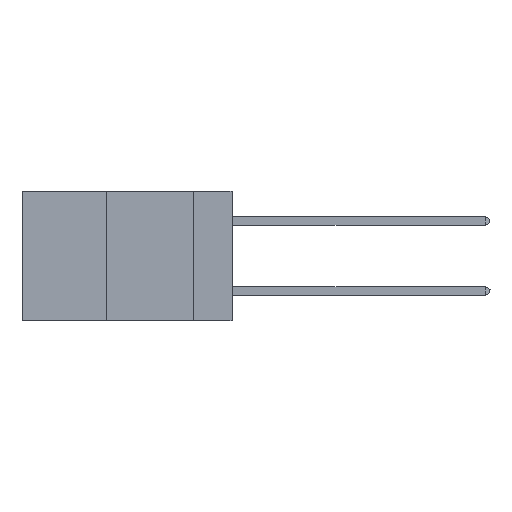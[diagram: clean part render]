
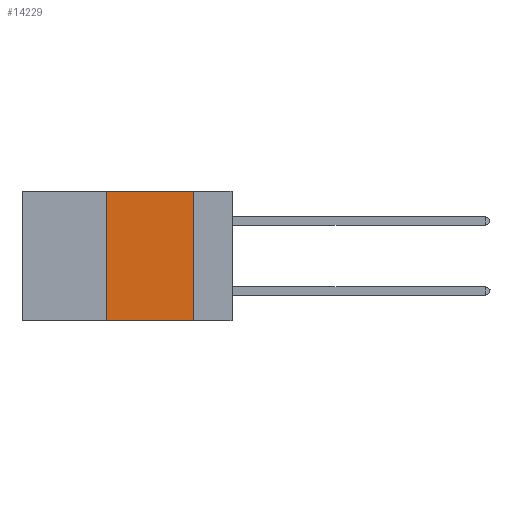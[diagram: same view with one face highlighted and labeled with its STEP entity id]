
A CAD part, left-side view. The second image highlights one B-rep face of the part: STEP entity #14229.
In plain terms, the highlighted planar face has unit normal (-1, 0, 0).
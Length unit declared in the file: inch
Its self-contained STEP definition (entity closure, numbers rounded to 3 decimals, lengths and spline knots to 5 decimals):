
#231 = DIRECTION ( 'NONE',  ( 0., -1., 0. ) ) ;
#595 = CARTESIAN_POINT ( 'NONE',  ( 0., 0.36, -0.37 ) ) ;
#899 = CARTESIAN_POINT ( 'NONE',  ( 0., 0.11, 0. ) ) ;
#1291 = DIRECTION ( 'NONE',  ( 0., 0., 1. ) ) ;
#1660 = VERTEX_POINT ( 'NONE', #8395 ) ;
#2934 = LINE ( 'NONE', #7076, #9794 ) ;
#3061 = EDGE_CURVE ( 'NONE', #1660, #17564, #10608, .T. ) ;
#4936 = CARTESIAN_POINT ( 'NONE',  ( 0., 0.36, 0. ) ) ;
#5480 = LINE ( 'NONE', #14958, #6207 ) ;
#6207 = VECTOR ( 'NONE', #12471, 39.37008 ) ;
#6398 = DIRECTION ( 'NONE',  ( 0., 0., -1. ) ) ;
#6500 = DIRECTION ( 'NONE',  ( 1., 0., 0. ) ) ;
#7076 = CARTESIAN_POINT ( 'NONE',  ( 0., 0.6, -0.37 ) ) ;
#7523 = ORIENTED_EDGE ( 'NONE', *, *, #7615, .T. ) ;
#7615 = EDGE_CURVE ( 'NONE', #10805, #17564, #2934, .T. ) ;
#7930 = FACE_OUTER_BOUND ( 'NONE', #8690, .T. ) ;
#8210 = LINE ( 'NONE', #10807, #11581 ) ;
#8395 = CARTESIAN_POINT ( 'NONE',  ( 0., 0.11, 0. ) ) ;
#8690 = EDGE_LOOP ( 'NONE', ( #16085, #14209, #10103, #7523 ) ) ;
#9794 = VECTOR ( 'NONE', #231, 39.37008 ) ;
#10103 = ORIENTED_EDGE ( 'NONE', *, *, #12572, .F. ) ;
#10608 = LINE ( 'NONE', #899, #15572 ) ;
#10805 = VERTEX_POINT ( 'NONE', #595 ) ;
#10807 = CARTESIAN_POINT ( 'NONE',  ( 0., 0.36, 0. ) ) ;
#10818 = CARTESIAN_POINT ( 'NONE',  ( 0., 0.11, -0.37 ) ) ;
#11581 = VECTOR ( 'NONE', #1291, 39.37008 ) ;
#12471 = DIRECTION ( 'NONE',  ( 0., -1., 0. ) ) ;
#12572 = EDGE_CURVE ( 'NONE', #10805, #14690, #8210, .T. ) ;
#14209 = ORIENTED_EDGE ( 'NONE', *, *, #14875, .F. ) ;
#14229 = ADVANCED_FACE ( 'NONE', ( #7930 ), #14808, .F. ) ;
#14478 = AXIS2_PLACEMENT_3D ( 'NONE', #15897, #6500, #17527 ) ;
#14690 = VERTEX_POINT ( 'NONE', #4936 ) ;
#14808 = PLANE ( 'NONE',  #14478 ) ;
#14875 = EDGE_CURVE ( 'NONE', #14690, #1660, #5480, .T. ) ;
#14958 = CARTESIAN_POINT ( 'NONE',  ( 0., 0.6, 0. ) ) ;
#15572 = VECTOR ( 'NONE', #6398, 39.37008 ) ;
#15897 = CARTESIAN_POINT ( 'NONE',  ( 0., 0.6, 0. ) ) ;
#16085 = ORIENTED_EDGE ( 'NONE', *, *, #3061, .F. ) ;
#17527 = DIRECTION ( 'NONE',  ( 0., 0., -1. ) ) ;
#17564 = VERTEX_POINT ( 'NONE', #10818 ) ;
